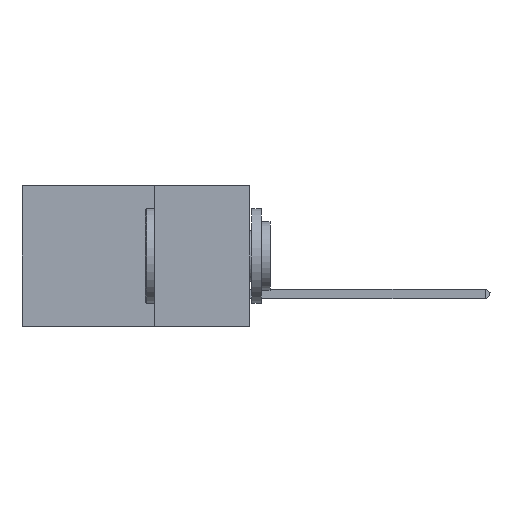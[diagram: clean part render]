
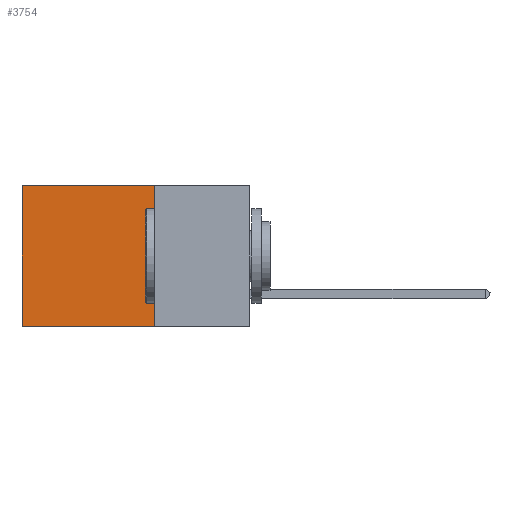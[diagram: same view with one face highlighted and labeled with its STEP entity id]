
A CAD part, left-side view. The second image highlights one B-rep face of the part: STEP entity #3754.
In plain terms, the highlighted planar face has unit normal (-1, 0, 0).
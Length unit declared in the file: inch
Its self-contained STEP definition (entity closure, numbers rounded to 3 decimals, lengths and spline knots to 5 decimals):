
#325 = LINE ( 'NONE', #17563, #14678 ) ;
#1108 = VERTEX_POINT ( 'NONE', #35870 ) ;
#3754 = ADVANCED_FACE ( 'NONE', ( #18098 ), #35479, .F. ) ;
#4004 = AXIS2_PLACEMENT_3D ( 'NONE', #39840, #24049, #20726 ) ;
#6544 = EDGE_CURVE ( 'NONE', #25309, #31103, #13657, .T. ) ;
#8302 = EDGE_CURVE ( 'NONE', #26379, #31103, #325, .T. ) ;
#8855 = VECTOR ( 'NONE', #26992, 39.37008 ) ;
#12515 = EDGE_CURVE ( 'NONE', #1108, #25309, #44186, .T. ) ;
#13617 = ORIENTED_EDGE ( 'NONE', *, *, #12515, .F. ) ;
#13657 = LINE ( 'NONE', #15159, #8855 ) ;
#14678 = VECTOR ( 'NONE', #24896, 39.37008 ) ;
#15159 = CARTESIAN_POINT ( 'NONE',  ( 0.2875, 0.25, -0.37 ) ) ;
#17563 = CARTESIAN_POINT ( 'NONE',  ( 0.2875, 0.6, 0. ) ) ;
#18098 = FACE_OUTER_BOUND ( 'NONE', #34806, .T. ) ;
#20726 = DIRECTION ( 'NONE',  ( 0., 0., -1. ) ) ;
#20838 = VECTOR ( 'NONE', #30245, 39.37008 ) ;
#21480 = CARTESIAN_POINT ( 'NONE',  ( 0.2875, 0.25, -0.37 ) ) ;
#24049 = DIRECTION ( 'NONE',  ( 1., 0., 0. ) ) ;
#24896 = DIRECTION ( 'NONE',  ( 0., 0., -1. ) ) ;
#24934 = LINE ( 'NONE', #38479, #43531 ) ;
#25309 = VERTEX_POINT ( 'NONE', #21480 ) ;
#26379 = VERTEX_POINT ( 'NONE', #27544 ) ;
#26992 = DIRECTION ( 'NONE',  ( 0., 1., 0. ) ) ;
#27544 = CARTESIAN_POINT ( 'NONE',  ( 0.2875, 0.6, 0. ) ) ;
#27978 = ORIENTED_EDGE ( 'NONE', *, *, #6544, .F. ) ;
#30245 = DIRECTION ( 'NONE',  ( 0., 0., -1. ) ) ;
#30798 = EDGE_CURVE ( 'NONE', #1108, #26379, #24934, .T. ) ;
#31103 = VERTEX_POINT ( 'NONE', #36100 ) ;
#34806 = EDGE_LOOP ( 'NONE', ( #39695, #27978, #13617, #45478 ) ) ;
#35479 = PLANE ( 'NONE',  #4004 ) ;
#35870 = CARTESIAN_POINT ( 'NONE',  ( 0.2875, 0.25, 0. ) ) ;
#36100 = CARTESIAN_POINT ( 'NONE',  ( 0.2875, 0.6, -0.37 ) ) ;
#38479 = CARTESIAN_POINT ( 'NONE',  ( 0.2875, 0.25, 0. ) ) ;
#39695 = ORIENTED_EDGE ( 'NONE', *, *, #8302, .T. ) ;
#39840 = CARTESIAN_POINT ( 'NONE',  ( 0.2875, 0.25, 0. ) ) ;
#41993 = DIRECTION ( 'NONE',  ( 0., 1., 0. ) ) ;
#43531 = VECTOR ( 'NONE', #41993, 39.37008 ) ;
#44186 = LINE ( 'NONE', #44881, #20838 ) ;
#44881 = CARTESIAN_POINT ( 'NONE',  ( 0.2875, 0.25, 0. ) ) ;
#45478 = ORIENTED_EDGE ( 'NONE', *, *, #30798, .T. ) ;
